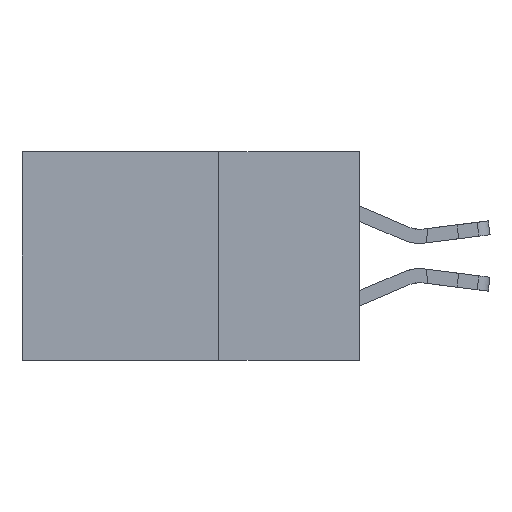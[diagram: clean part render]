
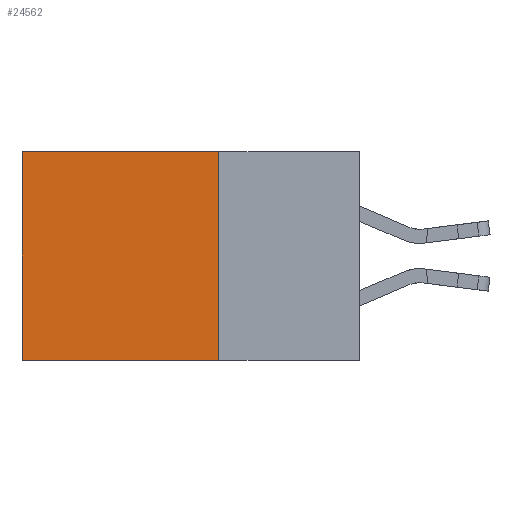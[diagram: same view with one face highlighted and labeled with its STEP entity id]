
A CAD part, left-side view. The second image highlights one B-rep face of the part: STEP entity #24562.
In plain terms, the highlighted planar face has unit normal (-1, 0, 0).
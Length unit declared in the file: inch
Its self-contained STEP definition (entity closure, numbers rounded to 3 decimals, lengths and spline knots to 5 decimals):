
#2354 = CARTESIAN_POINT ( 'NONE',  ( 0.2875, 0.25, 0. ) ) ;
#3811 = ORIENTED_EDGE ( 'NONE', *, *, #9410, .T. ) ;
#4435 = LINE ( 'NONE', #11418, #24714 ) ;
#4442 = LINE ( 'NONE', #4874, #20194 ) ;
#4874 = CARTESIAN_POINT ( 'NONE',  ( 0.2875, 0.25, -0.37 ) ) ;
#5616 = VERTEX_POINT ( 'NONE', #23171 ) ;
#6207 = CARTESIAN_POINT ( 'NONE',  ( 0.2875, 0.25, 0. ) ) ;
#7251 = EDGE_CURVE ( 'NONE', #5616, #20431, #14132, .T. ) ;
#7630 = VECTOR ( 'NONE', #14074, 39.37008 ) ;
#8155 = DIRECTION ( 'NONE',  ( 1., 0., 0. ) ) ;
#8472 = VECTOR ( 'NONE', #19805, 39.37008 ) ;
#9293 = EDGE_LOOP ( 'NONE', ( #3811, #9714, #11020, #20601 ) ) ;
#9410 = EDGE_CURVE ( 'NONE', #11074, #13458, #4435, .T. ) ;
#9714 = ORIENTED_EDGE ( 'NONE', *, *, #25049, .F. ) ;
#10048 = AXIS2_PLACEMENT_3D ( 'NONE', #2354, #8155, #16190 ) ;
#11020 = ORIENTED_EDGE ( 'NONE', *, *, #7251, .F. ) ;
#11074 = VERTEX_POINT ( 'NONE', #15121 ) ;
#11418 = CARTESIAN_POINT ( 'NONE',  ( 0.2875, 0.6, 0. ) ) ;
#12524 = EDGE_CURVE ( 'NONE', #5616, #11074, #17102, .T. ) ;
#13458 = VERTEX_POINT ( 'NONE', #19894 ) ;
#14074 = DIRECTION ( 'NONE',  ( 0., 0., -1. ) ) ;
#14114 = PLANE ( 'NONE',  #10048 ) ;
#14132 = LINE ( 'NONE', #6207, #7630 ) ;
#14349 = FACE_OUTER_BOUND ( 'NONE', #9293, .T. ) ;
#15121 = CARTESIAN_POINT ( 'NONE',  ( 0.2875, 0.6, 0. ) ) ;
#16190 = DIRECTION ( 'NONE',  ( 0., 0., -1. ) ) ;
#17102 = LINE ( 'NONE', #21704, #8472 ) ;
#17617 = DIRECTION ( 'NONE',  ( 0., 0., -1. ) ) ;
#18835 = CARTESIAN_POINT ( 'NONE',  ( 0.2875, 0.25, -0.37 ) ) ;
#18854 = DIRECTION ( 'NONE',  ( 0., 1., 0. ) ) ;
#19805 = DIRECTION ( 'NONE',  ( 0., 1., 0. ) ) ;
#19894 = CARTESIAN_POINT ( 'NONE',  ( 0.2875, 0.6, -0.37 ) ) ;
#20194 = VECTOR ( 'NONE', #18854, 39.37008 ) ;
#20431 = VERTEX_POINT ( 'NONE', #18835 ) ;
#20601 = ORIENTED_EDGE ( 'NONE', *, *, #12524, .T. ) ;
#21704 = CARTESIAN_POINT ( 'NONE',  ( 0.2875, 0.25, 0. ) ) ;
#23171 = CARTESIAN_POINT ( 'NONE',  ( 0.2875, 0.25, 0. ) ) ;
#24562 = ADVANCED_FACE ( 'NONE', ( #14349 ), #14114, .F. ) ;
#24714 = VECTOR ( 'NONE', #17617, 39.37008 ) ;
#25049 = EDGE_CURVE ( 'NONE', #20431, #13458, #4442, .T. ) ;
